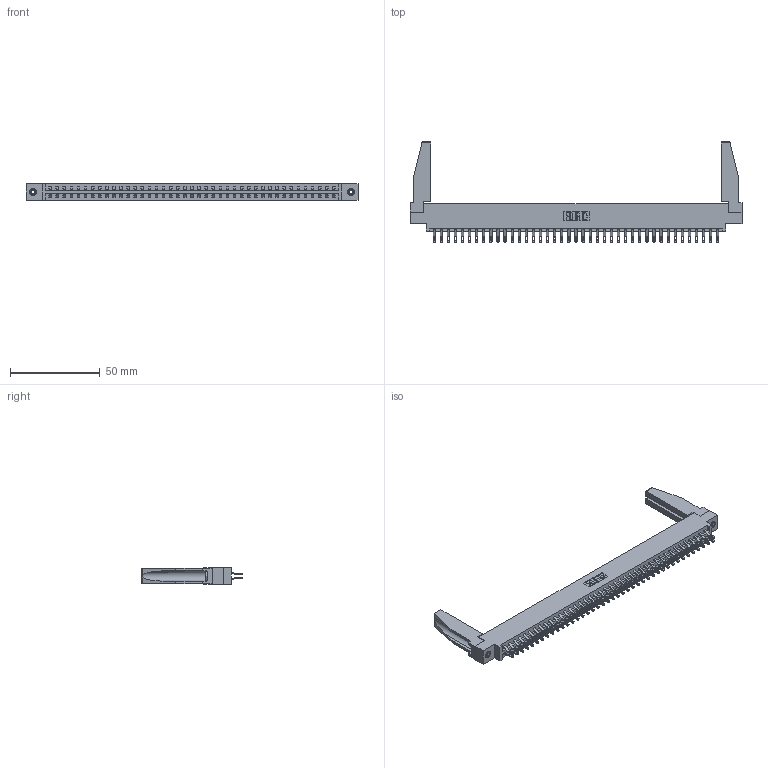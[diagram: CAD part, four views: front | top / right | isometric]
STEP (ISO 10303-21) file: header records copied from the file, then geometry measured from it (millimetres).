
FILE_DESCRIPTION (( 'STEP AP203' ), '1' );
FILE_NAME ('387-082-555-878.STEP', '2019-10-23T00:12:02', ( '' ), ( '' ), 'SwSTEP 2.0', 'SolidWorks 2016', '' );
FILE_SCHEMA (( 'CONFIG_CONTROL_DESIGN' ));
Length unit declared in the file: inch
Products named in the file (5): 337 Part_0.170 Offset - 0.156 Dia-TI; 307-220-078; 345-250-001_345-250-001-102; 345-292-001_555 Tail; 387-082-555-878
Assembly tree (87 placements, depth 2):
  387-082-555-878
    337 Part_0.170 Offset - 0.156 Dia-TI
    345-292-001_555 Tail  x82
    345-250-001_345-250-001-102  x2
    307-220-078  x2
Bounding box: 185.47 x 56.27 x 9.4 mm (x, y, z)
Volume: 23646.7 mm3; surface area: 27043.1 mm2
Topology: 87 solids, 87 shells, 5168 faces, 16151 edges, 10758 vertices
Faces by surface type: plane 3110, cylinder 2042, cone 12, torus 4
Entity records: 34816 total; most frequent: CARTESIAN_POINT 5902, ORIENTED_EDGE 5764, DIRECTION 4998, EDGE_CURVE 2882, LINE 2696, VECTOR 2696, VERTEX_POINT 1916, AXIS2_PLACEMENT_3D 1151
